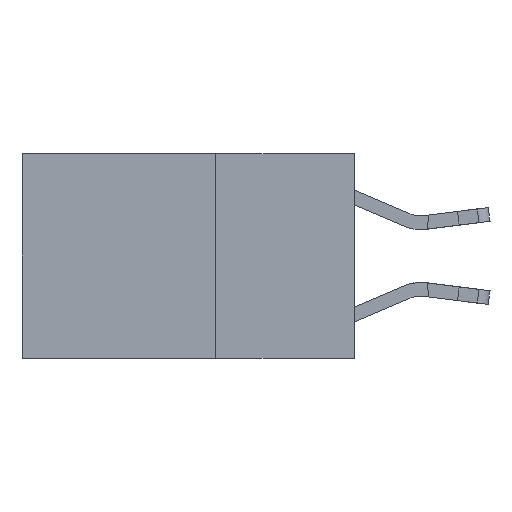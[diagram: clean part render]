
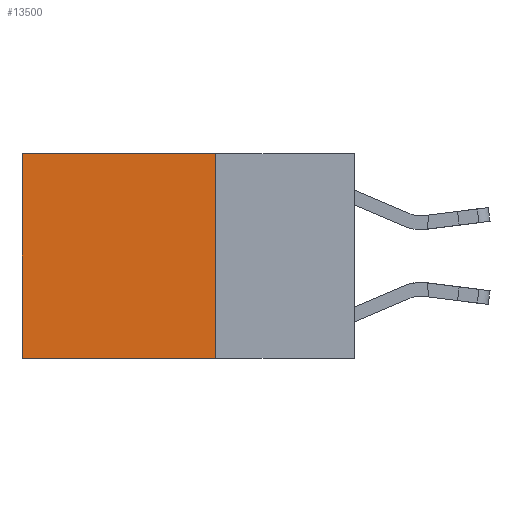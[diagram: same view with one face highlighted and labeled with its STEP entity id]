
A CAD part, left-side view. The second image highlights one B-rep face of the part: STEP entity #13500.
In plain terms, the highlighted planar face has unit normal (-1, 0, 0).
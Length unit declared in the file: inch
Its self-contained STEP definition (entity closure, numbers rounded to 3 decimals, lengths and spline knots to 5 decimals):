
#270 = LINE ( 'NONE', #3016, #26053 ) ;
#341 = LINE ( 'NONE', #27086, #13279 ) ;
#1556 = CARTESIAN_POINT ( 'NONE',  ( 0.2625, 0.25, 0. ) ) ;
#3016 = CARTESIAN_POINT ( 'NONE',  ( 0.2625, 0.25, 0. ) ) ;
#3674 = DIRECTION ( 'NONE',  ( 0., 0., -1. ) ) ;
#4488 = DIRECTION ( 'NONE',  ( 0., 1., 0. ) ) ;
#4717 = VERTEX_POINT ( 'NONE', #8960 ) ;
#4780 = VECTOR ( 'NONE', #4488, 39.37008 ) ;
#4923 = VECTOR ( 'NONE', #3674, 39.37008 ) ;
#5082 = DIRECTION ( 'NONE',  ( 1., 0., 0. ) ) ;
#6686 = EDGE_CURVE ( 'NONE', #26118, #21656, #27822, .T. ) ;
#6788 = LINE ( 'NONE', #24403, #4780 ) ;
#7976 = CARTESIAN_POINT ( 'NONE',  ( 0.2625, 0.25, 0. ) ) ;
#8194 = ORIENTED_EDGE ( 'NONE', *, *, #25888, .F. ) ;
#8619 = ORIENTED_EDGE ( 'NONE', *, *, #16307, .F. ) ;
#8960 = CARTESIAN_POINT ( 'NONE',  ( 0.2625, 0.25, -0.37 ) ) ;
#9774 = CARTESIAN_POINT ( 'NONE',  ( 0.2625, 0.6, 0. ) ) ;
#10204 = CARTESIAN_POINT ( 'NONE',  ( 0.2625, 0.6, 0. ) ) ;
#10750 = EDGE_LOOP ( 'NONE', ( #19275, #8194, #8619, #16076 ) ) ;
#10949 = DIRECTION ( 'NONE',  ( 0., 1., 0. ) ) ;
#11452 = DIRECTION ( 'NONE',  ( 0., 0., -1. ) ) ;
#11560 = CARTESIAN_POINT ( 'NONE',  ( 0.2625, 0.6, -0.37 ) ) ;
#13279 = VECTOR ( 'NONE', #10949, 39.37008 ) ;
#13500 = ADVANCED_FACE ( 'NONE', ( #21194 ), #27908, .F. ) ;
#16076 = ORIENTED_EDGE ( 'NONE', *, *, #21060, .T. ) ;
#16307 = EDGE_CURVE ( 'NONE', #25182, #4717, #270, .T. ) ;
#19275 = ORIENTED_EDGE ( 'NONE', *, *, #6686, .T. ) ;
#21060 = EDGE_CURVE ( 'NONE', #25182, #26118, #6788, .T. ) ;
#21194 = FACE_OUTER_BOUND ( 'NONE', #10750, .T. ) ;
#21656 = VERTEX_POINT ( 'NONE', #11560 ) ;
#22806 = DIRECTION ( 'NONE',  ( 0., 0., -1. ) ) ;
#24403 = CARTESIAN_POINT ( 'NONE',  ( 0.2625, 0.25, 0. ) ) ;
#25094 = AXIS2_PLACEMENT_3D ( 'NONE', #7976, #5082, #22806 ) ;
#25182 = VERTEX_POINT ( 'NONE', #1556 ) ;
#25888 = EDGE_CURVE ( 'NONE', #4717, #21656, #341, .T. ) ;
#26053 = VECTOR ( 'NONE', #11452, 39.37008 ) ;
#26118 = VERTEX_POINT ( 'NONE', #10204 ) ;
#27086 = CARTESIAN_POINT ( 'NONE',  ( 0.2625, 0.25, -0.37 ) ) ;
#27822 = LINE ( 'NONE', #9774, #4923 ) ;
#27908 = PLANE ( 'NONE',  #25094 ) ;
